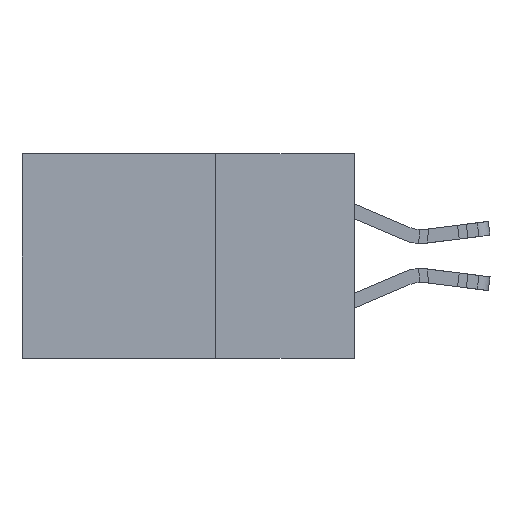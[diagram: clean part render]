
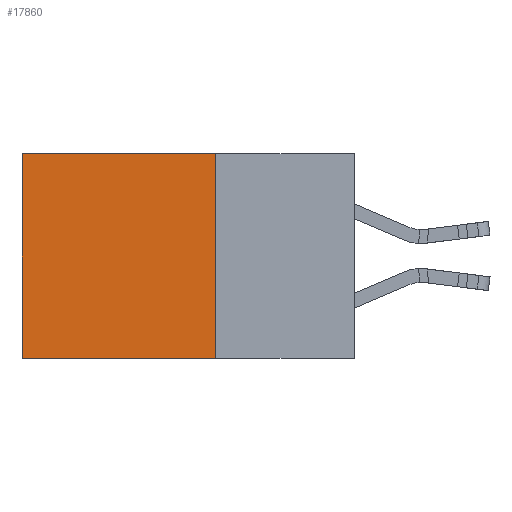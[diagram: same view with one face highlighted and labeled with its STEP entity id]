
A CAD part, left-side view. The second image highlights one B-rep face of the part: STEP entity #17860.
In plain terms, the highlighted planar face has unit normal (-1, 0, 0).
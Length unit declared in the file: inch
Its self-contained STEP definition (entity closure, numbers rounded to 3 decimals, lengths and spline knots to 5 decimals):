
#162 = CARTESIAN_POINT ( 'NONE',  ( 0.2615, 0.25, -0.37 ) ) ;
#438 = EDGE_CURVE ( 'NONE', #8591, #22895, #21589, .T. ) ;
#496 = DIRECTION ( 'NONE',  ( 0., 1., 0. ) ) ;
#528 = CARTESIAN_POINT ( 'NONE',  ( 0.2615, 0.25, 0. ) ) ;
#666 = DIRECTION ( 'NONE',  ( 0., 1., 0. ) ) ;
#1123 = DIRECTION ( 'NONE',  ( 1., 0., 0. ) ) ;
#1590 = EDGE_CURVE ( 'NONE', #22895, #7570, #21901, .T. ) ;
#2242 = FACE_OUTER_BOUND ( 'NONE', #12605, .T. ) ;
#3037 = VECTOR ( 'NONE', #496, 39.37008 ) ;
#4221 = EDGE_CURVE ( 'NONE', #8591, #21345, #17873, .T. ) ;
#7570 = VERTEX_POINT ( 'NONE', #9669 ) ;
#8591 = VERTEX_POINT ( 'NONE', #16513 ) ;
#9214 = ORIENTED_EDGE ( 'NONE', *, *, #4221, .T. ) ;
#9384 = ORIENTED_EDGE ( 'NONE', *, *, #22163, .T. ) ;
#9669 = CARTESIAN_POINT ( 'NONE',  ( 0.2615, 0.6, -0.37 ) ) ;
#12605 = EDGE_LOOP ( 'NONE', ( #9384, #17769, #16171, #9214 ) ) ;
#12613 = CARTESIAN_POINT ( 'NONE',  ( 0.2615, 0.25, -0.37 ) ) ;
#12636 = AXIS2_PLACEMENT_3D ( 'NONE', #12613, #1123, #14652 ) ;
#12694 = PLANE ( 'NONE',  #12636 ) ;
#14652 = DIRECTION ( 'NONE',  ( 0., 0., -1. ) ) ;
#16171 = ORIENTED_EDGE ( 'NONE', *, *, #438, .F. ) ;
#16507 = VECTOR ( 'NONE', #22949, 39.37008 ) ;
#16513 = CARTESIAN_POINT ( 'NONE',  ( 0.2615, 0.25, 0. ) ) ;
#17043 = DIRECTION ( 'NONE',  ( 0., 0., -1. ) ) ;
#17419 = VECTOR ( 'NONE', #666, 39.37008 ) ;
#17769 = ORIENTED_EDGE ( 'NONE', *, *, #1590, .F. ) ;
#17860 = ADVANCED_FACE ( 'NONE', ( #2242 ), #12694, .F. ) ;
#17873 = LINE ( 'NONE', #528, #3037 ) ;
#20333 = VECTOR ( 'NONE', #17043, 39.37008 ) ;
#20920 = LINE ( 'NONE', #22726, #20333 ) ;
#20923 = CARTESIAN_POINT ( 'NONE',  ( 0.2615, 0.25, -0.37 ) ) ;
#21345 = VERTEX_POINT ( 'NONE', #22340 ) ;
#21589 = LINE ( 'NONE', #22795, #16507 ) ;
#21901 = LINE ( 'NONE', #162, #17419 ) ;
#22163 = EDGE_CURVE ( 'NONE', #21345, #7570, #20920, .T. ) ;
#22340 = CARTESIAN_POINT ( 'NONE',  ( 0.2615, 0.6, 0. ) ) ;
#22726 = CARTESIAN_POINT ( 'NONE',  ( 0.2615, 0.6, -0.37 ) ) ;
#22795 = CARTESIAN_POINT ( 'NONE',  ( 0.2615, 0.25, -0.37 ) ) ;
#22895 = VERTEX_POINT ( 'NONE', #20923 ) ;
#22949 = DIRECTION ( 'NONE',  ( 0., 0., -1. ) ) ;
